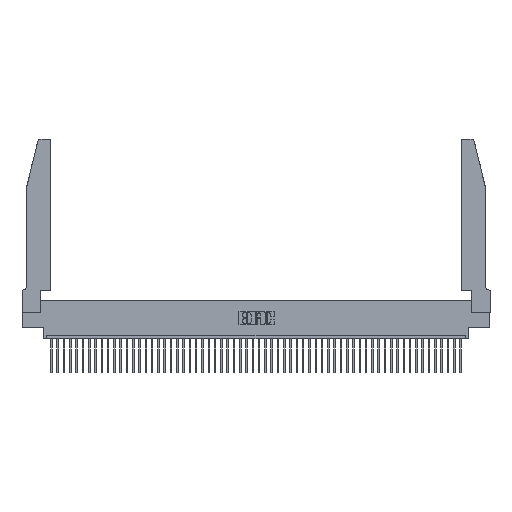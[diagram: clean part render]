
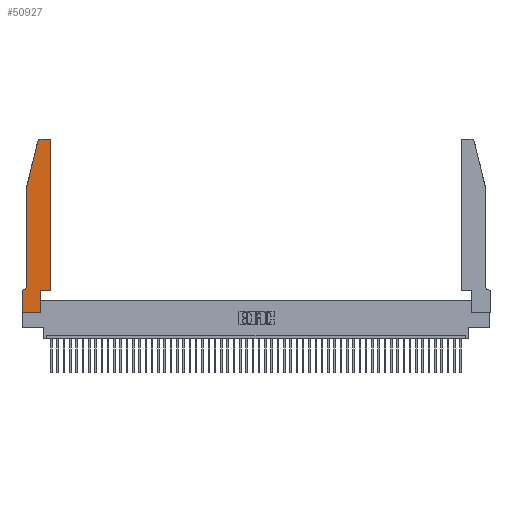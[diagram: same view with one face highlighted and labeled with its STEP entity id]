
A CAD part, top view. The second image highlights one B-rep face of the part: STEP entity #50927.
In plain terms, the highlighted planar face has unit normal (0, 0, 1).
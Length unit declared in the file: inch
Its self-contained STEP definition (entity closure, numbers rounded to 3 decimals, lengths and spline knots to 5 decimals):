
#143 = ORIENTED_EDGE ( 'NONE', *, *, #48256, .T. ) ;
#232 = EDGE_CURVE ( 'NONE', #42795, #23752, #47036, .T. ) ;
#284 = CARTESIAN_POINT ( 'NONE',  ( 0.284, 2.75, 0.37 ) ) ;
#395 = CARTESIAN_POINT ( 'NONE',  ( 0.4505, 2.72, 0.37 ) ) ;
#983 = ORIENTED_EDGE ( 'NONE', *, *, #42578, .T. ) ;
#1092 = CARTESIAN_POINT ( 'NONE',  ( 0.0755, 2., 0.37 ) ) ;
#1566 = DIRECTION ( 'NONE',  ( 0., 0., 1. ) ) ;
#2647 = EDGE_LOOP ( 'NONE', ( #39263, #48209, #19662, #8587, #41935, #28639, #8502, #143, #983, #8522, #44862, #45708 ) ) ;
#2874 = DIRECTION ( 'NONE',  ( 0., 1., 0. ) ) ;
#3078 = VECTOR ( 'NONE', #13666, 39.37008 ) ;
#3974 = EDGE_CURVE ( 'NONE', #31161, #32547, #11067, .T. ) ;
#4310 = VECTOR ( 'NONE', #44817, 39.37008 ) ;
#4824 = VECTOR ( 'NONE', #40016, 39.37008 ) ;
#5274 = DIRECTION ( 'NONE',  ( 1., 0., 0. ) ) ;
#6113 = VECTOR ( 'NONE', #32119, 39.37008 ) ;
#6909 = CARTESIAN_POINT ( 'NONE',  ( 0.4205, 2.75, 0.37 ) ) ;
#8020 = VERTEX_POINT ( 'NONE', #32661 ) ;
#8502 = ORIENTED_EDGE ( 'NONE', *, *, #18641, .T. ) ;
#8522 = ORIENTED_EDGE ( 'NONE', *, *, #9946, .T. ) ;
#8587 = ORIENTED_EDGE ( 'NONE', *, *, #44666, .T. ) ;
#8908 = DIRECTION ( 'NONE',  ( -1., 0., 0. ) ) ;
#9130 = CARTESIAN_POINT ( 'NONE',  ( 0.4205, 2.72, 0.37 ) ) ;
#9946 = EDGE_CURVE ( 'NONE', #38403, #19864, #26773, .T. ) ;
#10019 = VECTOR ( 'NONE', #5274, 39.37008 ) ;
#11067 = LINE ( 'NONE', #20189, #6113 ) ;
#11551 = CARTESIAN_POINT ( 'NONE',  ( 0.0055, 0.42, 0.37 ) ) ;
#12795 = CARTESIAN_POINT ( 'NONE',  ( 0., 0.35, 0.37 ) ) ;
#13495 = CARTESIAN_POINT ( 'NONE',  ( 0.2865, 0.35, 0.37 ) ) ;
#13666 = DIRECTION ( 'NONE',  ( 0., 1., 0. ) ) ;
#13898 = VERTEX_POINT ( 'NONE', #22420 ) ;
#14814 = LINE ( 'NONE', #28183, #4310 ) ;
#16522 = DIRECTION ( 'NONE',  ( 0., 0., 1. ) ) ;
#17126 = CIRCLE ( 'NONE', #28263, 0.07 ) ;
#18641 = EDGE_CURVE ( 'NONE', #22072, #13898, #26299, .T. ) ;
#19350 = CIRCLE ( 'NONE', #31123, 0.03 ) ;
#19662 = ORIENTED_EDGE ( 'NONE', *, *, #232, .T. ) ;
#19864 = VERTEX_POINT ( 'NONE', #45244 ) ;
#20126 = AXIS2_PLACEMENT_3D ( 'NONE', #9130, #16522, #44434 ) ;
#20189 = CARTESIAN_POINT ( 'NONE',  ( 0.2605, 2.75, 0.37 ) ) ;
#20764 = FACE_OUTER_BOUND ( 'NONE', #2647, .T. ) ;
#20950 = AXIS2_PLACEMENT_3D ( 'NONE', #12795, #1566, #40487 ) ;
#21755 = CARTESIAN_POINT ( 'NONE',  ( 0.284, 2.72, 0.37 ) ) ;
#22072 = VERTEX_POINT ( 'NONE', #39898 ) ;
#22420 = CARTESIAN_POINT ( 'NONE',  ( 0., 0., 0.37 ) ) ;
#23752 = VERTEX_POINT ( 'NONE', #33263 ) ;
#23812 = LINE ( 'NONE', #40799, #41816 ) ;
#24952 = CARTESIAN_POINT ( 'NONE',  ( 0.0755, 0.35, 0.37 ) ) ;
#25752 = CARTESIAN_POINT ( 'NONE',  ( 0.25487, 2.72718, 0.37 ) ) ;
#25770 = DIRECTION ( 'NONE',  ( 1., 0., 0. ) ) ;
#25871 = DIRECTION ( 'NONE',  ( 0., -1., 0. ) ) ;
#26035 = CARTESIAN_POINT ( 'NONE',  ( 0., 0., 0.37 ) ) ;
#26299 = LINE ( 'NONE', #26035, #33036 ) ;
#26773 = LINE ( 'NONE', #49256, #10019 ) ;
#28183 = CARTESIAN_POINT ( 'NONE',  ( 0., 0., 0.37 ) ) ;
#28263 = AXIS2_PLACEMENT_3D ( 'NONE', #11551, #30897, #35229 ) ;
#28639 = ORIENTED_EDGE ( 'NONE', *, *, #45351, .T. ) ;
#29355 = CIRCLE ( 'NONE', #20126, 0.03 ) ;
#30649 = VECTOR ( 'NONE', #8908, 39.37008 ) ;
#30897 = DIRECTION ( 'NONE',  ( 0., 0., -1. ) ) ;
#31123 = AXIS2_PLACEMENT_3D ( 'NONE', #21755, #49517, #25770 ) ;
#31161 = VERTEX_POINT ( 'NONE', #6909 ) ;
#31245 = LINE ( 'NONE', #38270, #51182 ) ;
#31667 = EDGE_CURVE ( 'NONE', #19864, #47504, #31245, .T. ) ;
#32119 = DIRECTION ( 'NONE',  ( -1., 0., 0. ) ) ;
#32547 = VERTEX_POINT ( 'NONE', #284 ) ;
#32661 = CARTESIAN_POINT ( 'NONE',  ( 0.2865, 0., 0.37 ) ) ;
#33036 = VECTOR ( 'NONE', #25871, 39.37008 ) ;
#33263 = CARTESIAN_POINT ( 'NONE',  ( 0.0755, 2., 0.37 ) ) ;
#34018 = CARTESIAN_POINT ( 'NONE',  ( 0.0055, 0.35, 0.37 ) ) ;
#35229 = DIRECTION ( 'NONE',  ( -1., 0., 0. ) ) ;
#35404 = EDGE_CURVE ( 'NONE', #32547, #42795, #19350, .T. ) ;
#36476 = PLANE ( 'NONE',  #20950 ) ;
#38270 = CARTESIAN_POINT ( 'NONE',  ( 0.4505, 0.35, 0.37 ) ) ;
#38403 = VERTEX_POINT ( 'NONE', #38860 ) ;
#38406 = EDGE_CURVE ( 'NONE', #47300, #44842, #17126, .T. ) ;
#38860 = CARTESIAN_POINT ( 'NONE',  ( 0.2865, 0.35, 0.37 ) ) ;
#39263 = ORIENTED_EDGE ( 'NONE', *, *, #3974, .T. ) ;
#39897 = LINE ( 'NONE', #24952, #30649 ) ;
#39898 = CARTESIAN_POINT ( 'NONE',  ( 0., 0.35, 0.37 ) ) ;
#40016 = DIRECTION ( 'NONE',  ( -0.239, -0.971, 0. ) ) ;
#40487 = DIRECTION ( 'NONE',  ( 1., 0., 0. ) ) ;
#40799 = CARTESIAN_POINT ( 'NONE',  ( 0.0755, 2., 0.37 ) ) ;
#41816 = VECTOR ( 'NONE', #48131, 39.37008 ) ;
#41935 = ORIENTED_EDGE ( 'NONE', *, *, #38406, .T. ) ;
#42578 = EDGE_CURVE ( 'NONE', #8020, #38403, #47053, .T. ) ;
#42795 = VERTEX_POINT ( 'NONE', #25752 ) ;
#44434 = DIRECTION ( 'NONE',  ( 1., 0., 0. ) ) ;
#44572 = EDGE_CURVE ( 'NONE', #47504, #31161, #29355, .T. ) ;
#44666 = EDGE_CURVE ( 'NONE', #23752, #47300, #23812, .T. ) ;
#44817 = DIRECTION ( 'NONE',  ( 1., 0., 0. ) ) ;
#44842 = VERTEX_POINT ( 'NONE', #34018 ) ;
#44862 = ORIENTED_EDGE ( 'NONE', *, *, #31667, .T. ) ;
#45244 = CARTESIAN_POINT ( 'NONE',  ( 0.4505, 0.35, 0.37 ) ) ;
#45351 = EDGE_CURVE ( 'NONE', #44842, #22072, #39897, .T. ) ;
#45708 = ORIENTED_EDGE ( 'NONE', *, *, #44572, .T. ) ;
#47036 = LINE ( 'NONE', #1092, #4824 ) ;
#47053 = LINE ( 'NONE', #13495, #3078 ) ;
#47300 = VERTEX_POINT ( 'NONE', #50182 ) ;
#47504 = VERTEX_POINT ( 'NONE', #395 ) ;
#48131 = DIRECTION ( 'NONE',  ( 0., -1., 0. ) ) ;
#48209 = ORIENTED_EDGE ( 'NONE', *, *, #35404, .T. ) ;
#48256 = EDGE_CURVE ( 'NONE', #13898, #8020, #14814, .T. ) ;
#49256 = CARTESIAN_POINT ( 'NONE',  ( 0.4505, 0.35, 0.37 ) ) ;
#49517 = DIRECTION ( 'NONE',  ( 0., 0., 1. ) ) ;
#50182 = CARTESIAN_POINT ( 'NONE',  ( 0.0755, 0.42, 0.37 ) ) ;
#50927 = ADVANCED_FACE ( 'NONE', ( #20764 ), #36476, .T. ) ;
#51182 = VECTOR ( 'NONE', #2874, 39.37008 ) ;
